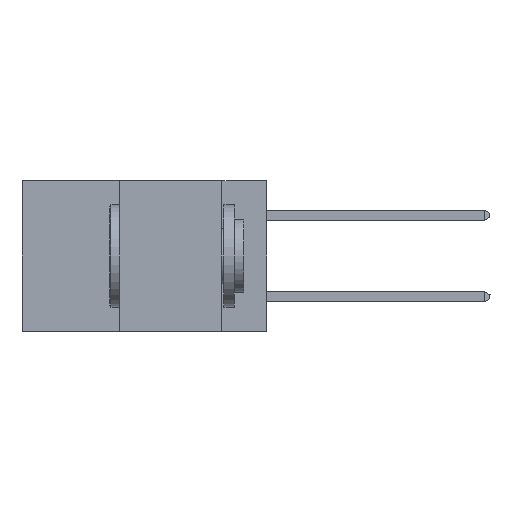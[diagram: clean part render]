
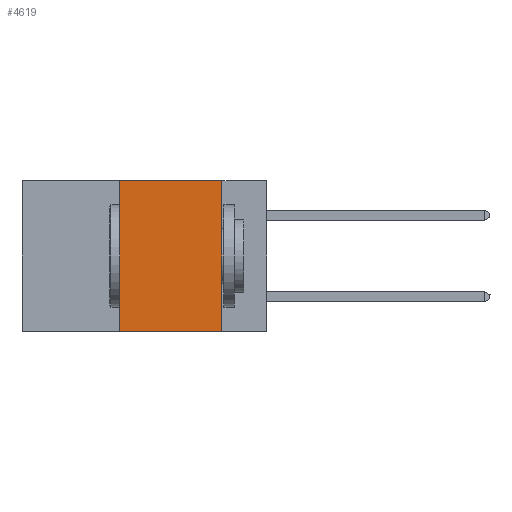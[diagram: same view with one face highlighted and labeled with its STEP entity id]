
A CAD part, left-side view. The second image highlights one B-rep face of the part: STEP entity #4619.
In plain terms, the highlighted planar face has unit normal (-1, 0, 0).
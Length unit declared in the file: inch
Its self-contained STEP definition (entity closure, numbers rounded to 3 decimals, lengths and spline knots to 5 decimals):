
#311 = DIRECTION ( 'NONE',  ( 0., -1., 0. ) ) ;
#1112 = ORIENTED_EDGE ( 'NONE', *, *, #21827, .F. ) ;
#1768 = DIRECTION ( 'NONE',  ( 0., 0., -1. ) ) ;
#2442 = PLANE ( 'NONE',  #6558 ) ;
#3357 = VECTOR ( 'NONE', #311, 39.37008 ) ;
#4322 = DIRECTION ( 'NONE',  ( 0., -1., 0. ) ) ;
#4599 = DIRECTION ( 'NONE',  ( 0., 0., -1. ) ) ;
#4619 = ADVANCED_FACE ( 'NONE', ( #7482 ), #2442, .F. ) ;
#5148 = VERTEX_POINT ( 'NONE', #7107 ) ;
#5588 = ORIENTED_EDGE ( 'NONE', *, *, #17305, .F. ) ;
#6035 = VECTOR ( 'NONE', #1768, 39.37008 ) ;
#6558 = AXIS2_PLACEMENT_3D ( 'NONE', #18060, #19823, #4599 ) ;
#6647 = EDGE_CURVE ( 'NONE', #5148, #16973, #11372, .T. ) ;
#7107 = CARTESIAN_POINT ( 'NONE',  ( 0., 0.11, 0. ) ) ;
#7482 = FACE_OUTER_BOUND ( 'NONE', #15794, .T. ) ;
#7518 = DIRECTION ( 'NONE',  ( 0., 0., 1. ) ) ;
#7547 = CARTESIAN_POINT ( 'NONE',  ( 0., 0.6, -0.37 ) ) ;
#8782 = CARTESIAN_POINT ( 'NONE',  ( 0., 0.6, 0. ) ) ;
#11124 = CARTESIAN_POINT ( 'NONE',  ( 0., 0.11, -0.37 ) ) ;
#11372 = LINE ( 'NONE', #13014, #6035 ) ;
#11984 = LINE ( 'NONE', #7547, #15920 ) ;
#13014 = CARTESIAN_POINT ( 'NONE',  ( 0., 0.11, 0. ) ) ;
#14236 = CARTESIAN_POINT ( 'NONE',  ( 0., 0.36, 0. ) ) ;
#15794 = EDGE_LOOP ( 'NONE', ( #17411, #5588, #1112, #18458 ) ) ;
#15920 = VECTOR ( 'NONE', #4322, 39.37008 ) ;
#16097 = LINE ( 'NONE', #8782, #3357 ) ;
#16973 = VERTEX_POINT ( 'NONE', #11124 ) ;
#17305 = EDGE_CURVE ( 'NONE', #20736, #5148, #16097, .T. ) ;
#17411 = ORIENTED_EDGE ( 'NONE', *, *, #6647, .F. ) ;
#17476 = LINE ( 'NONE', #14236, #21798 ) ;
#18060 = CARTESIAN_POINT ( 'NONE',  ( 0., 0.6, 0. ) ) ;
#18458 = ORIENTED_EDGE ( 'NONE', *, *, #21316, .T. ) ;
#19331 = CARTESIAN_POINT ( 'NONE',  ( 0., 0.36, -0.37 ) ) ;
#19823 = DIRECTION ( 'NONE',  ( 1., 0., 0. ) ) ;
#20723 = VERTEX_POINT ( 'NONE', #19331 ) ;
#20736 = VERTEX_POINT ( 'NONE', #21134 ) ;
#21134 = CARTESIAN_POINT ( 'NONE',  ( 0., 0.36, 0. ) ) ;
#21316 = EDGE_CURVE ( 'NONE', #20723, #16973, #11984, .T. ) ;
#21798 = VECTOR ( 'NONE', #7518, 39.37008 ) ;
#21827 = EDGE_CURVE ( 'NONE', #20723, #20736, #17476, .T. ) ;
